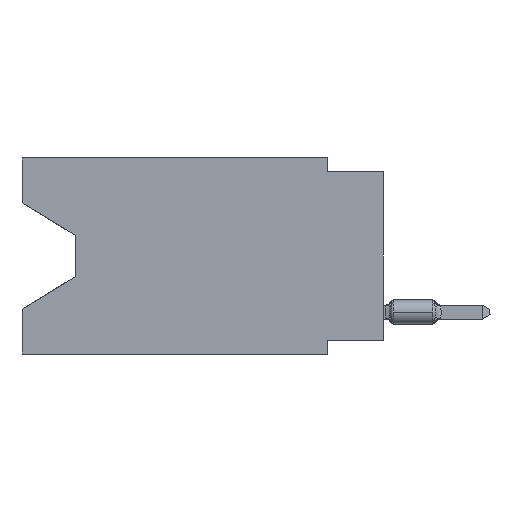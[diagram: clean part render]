
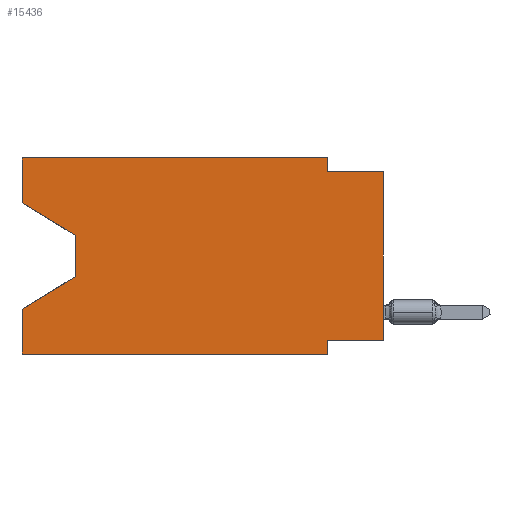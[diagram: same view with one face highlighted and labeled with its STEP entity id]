
A CAD part, left-side view. The second image highlights one B-rep face of the part: STEP entity #15436.
In plain terms, the highlighted planar face has unit normal (-1, 0, 0).
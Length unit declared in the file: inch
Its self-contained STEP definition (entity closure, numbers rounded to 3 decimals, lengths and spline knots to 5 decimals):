
#338 = VECTOR ( 'NONE', #30405, 39.37008 ) ;
#833 = CARTESIAN_POINT ( 'NONE',  ( 0., 0.1, -0.35 ) ) ;
#868 = VERTEX_POINT ( 'NONE', #14285 ) ;
#873 = ORIENTED_EDGE ( 'NONE', *, *, #5671, .F. ) ;
#947 = VECTOR ( 'NONE', #28132, 39.37008 ) ;
#1340 = CARTESIAN_POINT ( 'NONE',  ( 0., 0.645, 0. ) ) ;
#1414 = VECTOR ( 'NONE', #27559, 39.37008 ) ;
#1423 = CARTESIAN_POINT ( 'NONE',  ( 0., 0.1, 0. ) ) ;
#1795 = ORIENTED_EDGE ( 'NONE', *, *, #16061, .T. ) ;
#2090 = DIRECTION ( 'NONE',  ( 0., -1., 0. ) ) ;
#2519 = VECTOR ( 'NONE', #8801, 39.37008 ) ;
#2602 = DIRECTION ( 'NONE',  ( 0., 0., 1. ) ) ;
#2802 = EDGE_CURVE ( 'NONE', #32336, #28358, #22789, .T. ) ;
#2867 = VERTEX_POINT ( 'NONE', #30764 ) ;
#2875 = VECTOR ( 'NONE', #5446, 39.37008 ) ;
#3152 = EDGE_CURVE ( 'NONE', #7611, #32927, #6122, .T. ) ;
#3556 = CARTESIAN_POINT ( 'NONE',  ( 0., 0.55, -0.138 ) ) ;
#3608 = VERTEX_POINT ( 'NONE', #30514 ) ;
#3886 = DIRECTION ( 'NONE',  ( 0., 0., 1. ) ) ;
#4242 = EDGE_CURVE ( 'NONE', #10648, #868, #19215, .T. ) ;
#4525 = VECTOR ( 'NONE', #23194, 39.37008 ) ;
#5014 = LINE ( 'NONE', #17437, #947 ) ;
#5392 = EDGE_CURVE ( 'NONE', #18078, #32336, #28736, .T. ) ;
#5446 = DIRECTION ( 'NONE',  ( 0., 0., -1. ) ) ;
#5654 = ORIENTED_EDGE ( 'NONE', *, *, #24397, .F. ) ;
#5671 = EDGE_CURVE ( 'NONE', #868, #7469, #12565, .T. ) ;
#5937 = CARTESIAN_POINT ( 'NONE',  ( 0., 0., -0.025 ) ) ;
#6122 = LINE ( 'NONE', #833, #19167 ) ;
#6707 = ORIENTED_EDGE ( 'NONE', *, *, #21748, .F. ) ;
#6810 = DIRECTION ( 'NONE',  ( 1., 0., 0. ) ) ;
#7469 = VERTEX_POINT ( 'NONE', #1423 ) ;
#7611 = VERTEX_POINT ( 'NONE', #22837 ) ;
#8055 = CARTESIAN_POINT ( 'NONE',  ( 0., 0., -0.025 ) ) ;
#8103 = VECTOR ( 'NONE', #2602, 39.37008 ) ;
#8134 = EDGE_CURVE ( 'NONE', #3608, #7611, #21937, .T. ) ;
#8801 = DIRECTION ( 'NONE',  ( 0., -1., 0. ) ) ;
#9134 = DIRECTION ( 'NONE',  ( 0., 0., 1. ) ) ;
#9453 = ORIENTED_EDGE ( 'NONE', *, *, #4242, .F. ) ;
#9528 = VECTOR ( 'NONE', #3886, 39.37008 ) ;
#9778 = EDGE_CURVE ( 'NONE', #30153, #28358, #22052, .T. ) ;
#10648 = VERTEX_POINT ( 'NONE', #14921 ) ;
#11154 = CARTESIAN_POINT ( 'NONE',  ( 0., 0.645, -0.35 ) ) ;
#12028 = CARTESIAN_POINT ( 'NONE',  ( 0., 0.645, 0. ) ) ;
#12253 = VERTEX_POINT ( 'NONE', #5937 ) ;
#12565 = LINE ( 'NONE', #25289, #338 ) ;
#13319 = VECTOR ( 'NONE', #9134, 39.37008 ) ;
#13737 = CARTESIAN_POINT ( 'NONE',  ( 0., 0.645, -0.35 ) ) ;
#14285 = CARTESIAN_POINT ( 'NONE',  ( 0., 0.645, 0. ) ) ;
#14415 = CARTESIAN_POINT ( 'NONE',  ( 0., 0.55, -0.212 ) ) ;
#14921 = CARTESIAN_POINT ( 'NONE',  ( 0., 0.645, -0.08025 ) ) ;
#15208 = LINE ( 'NONE', #28455, #8103 ) ;
#15366 = CARTESIAN_POINT ( 'NONE',  ( 0., 0.1, -0.35 ) ) ;
#15436 = ADVANCED_FACE ( 'NONE', ( #22448 ), #30091, .F. ) ;
#16061 = EDGE_CURVE ( 'NONE', #30153, #32927, #16776, .T. ) ;
#16776 = LINE ( 'NONE', #13737, #2519 ) ;
#16847 = ORIENTED_EDGE ( 'NONE', *, *, #2802, .T. ) ;
#17437 = CARTESIAN_POINT ( 'NONE',  ( 0., 0.645, -0.08025 ) ) ;
#17631 = ORIENTED_EDGE ( 'NONE', *, *, #18482, .T. ) ;
#18078 = VERTEX_POINT ( 'NONE', #21698 ) ;
#18482 = EDGE_CURVE ( 'NONE', #3608, #12253, #15208, .T. ) ;
#18698 = DIRECTION ( 'NONE',  ( 0., 0., -1. ) ) ;
#19167 = VECTOR ( 'NONE', #18698, 39.37008 ) ;
#19215 = LINE ( 'NONE', #1340, #9528 ) ;
#19218 = DIRECTION ( 'NONE',  ( 0., 1., 0. ) ) ;
#19767 = ORIENTED_EDGE ( 'NONE', *, *, #29978, .T. ) ;
#21698 = CARTESIAN_POINT ( 'NONE',  ( 0., 0.55, -0.138 ) ) ;
#21748 = EDGE_CURVE ( 'NONE', #2867, #12253, #23519, .T. ) ;
#21751 = VECTOR ( 'NONE', #19218, 39.37008 ) ;
#21845 = AXIS2_PLACEMENT_3D ( 'NONE', #30253, #6810, #25140 ) ;
#21937 = LINE ( 'NONE', #29913, #21751 ) ;
#22052 = LINE ( 'NONE', #12028, #13319 ) ;
#22448 = FACE_OUTER_BOUND ( 'NONE', #33454, .T. ) ;
#22693 = CARTESIAN_POINT ( 'NONE',  ( 0., 0.1, 0. ) ) ;
#22789 = LINE ( 'NONE', #25163, #1414 ) ;
#22837 = CARTESIAN_POINT ( 'NONE',  ( 0., 0.1, -0.325 ) ) ;
#23194 = DIRECTION ( 'NONE',  ( 0., 0., -1. ) ) ;
#23365 = LINE ( 'NONE', #22693, #4525 ) ;
#23519 = LINE ( 'NONE', #8055, #26591 ) ;
#23895 = ORIENTED_EDGE ( 'NONE', *, *, #8134, .F. ) ;
#24155 = ORIENTED_EDGE ( 'NONE', *, *, #9778, .F. ) ;
#24397 = EDGE_CURVE ( 'NONE', #7469, #2867, #23365, .T. ) ;
#25140 = DIRECTION ( 'NONE',  ( 0., 0., -1. ) ) ;
#25163 = CARTESIAN_POINT ( 'NONE',  ( 0., 0.55, -0.212 ) ) ;
#25289 = CARTESIAN_POINT ( 'NONE',  ( 0., 0.645, 0. ) ) ;
#26591 = VECTOR ( 'NONE', #2090, 39.37008 ) ;
#27559 = DIRECTION ( 'NONE',  ( 0., 0.855, -0.519 ) ) ;
#27658 = CARTESIAN_POINT ( 'NONE',  ( 0., 0.645, -0.26975 ) ) ;
#28132 = DIRECTION ( 'NONE',  ( 0., -0.855, -0.519 ) ) ;
#28358 = VERTEX_POINT ( 'NONE', #27658 ) ;
#28455 = CARTESIAN_POINT ( 'NONE',  ( 0., 0., 0. ) ) ;
#28736 = LINE ( 'NONE', #3556, #2875 ) ;
#29634 = ORIENTED_EDGE ( 'NONE', *, *, #5392, .T. ) ;
#29913 = CARTESIAN_POINT ( 'NONE',  ( 0., 0., -0.325 ) ) ;
#29978 = EDGE_CURVE ( 'NONE', #10648, #18078, #5014, .T. ) ;
#30091 = PLANE ( 'NONE',  #21845 ) ;
#30153 = VERTEX_POINT ( 'NONE', #11154 ) ;
#30253 = CARTESIAN_POINT ( 'NONE',  ( 0., 0.645, 0. ) ) ;
#30405 = DIRECTION ( 'NONE',  ( 0., -1., 0. ) ) ;
#30514 = CARTESIAN_POINT ( 'NONE',  ( 0., 0., -0.325 ) ) ;
#30764 = CARTESIAN_POINT ( 'NONE',  ( 0., 0.1, -0.025 ) ) ;
#32336 = VERTEX_POINT ( 'NONE', #14415 ) ;
#32927 = VERTEX_POINT ( 'NONE', #15366 ) ;
#33055 = ORIENTED_EDGE ( 'NONE', *, *, #3152, .F. ) ;
#33454 = EDGE_LOOP ( 'NONE', ( #19767, #29634, #16847, #24155, #1795, #33055, #23895, #17631, #6707, #5654, #873, #9453 ) ) ;
